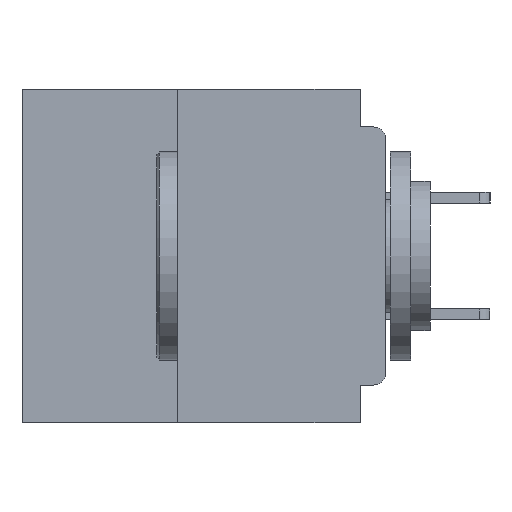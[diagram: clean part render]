
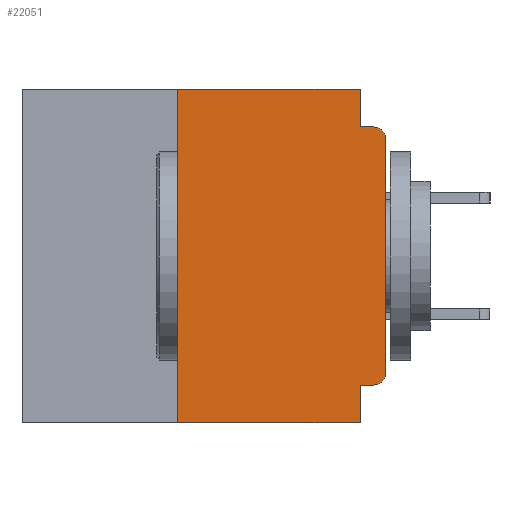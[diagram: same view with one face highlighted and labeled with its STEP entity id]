
A CAD part, left-side view. The second image highlights one B-rep face of the part: STEP entity #22051.
In plain terms, the highlighted planar face has unit normal (-1, 0, 0).
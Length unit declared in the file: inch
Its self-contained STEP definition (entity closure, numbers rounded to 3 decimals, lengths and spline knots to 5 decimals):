
#986 = ORIENTED_EDGE ( 'NONE', *, *, #8208, .F. ) ;
#1504 = EDGE_CURVE ( 'NONE', #35069, #13415, #29228, .T. ) ;
#2029 = VECTOR ( 'NONE', #14272, 39.37008 ) ;
#3005 = ORIENTED_EDGE ( 'NONE', *, *, #14251, .T. ) ;
#3397 = EDGE_LOOP ( 'NONE', ( #20141, #14638, #27694, #10907, #6797, #986, #3005, #25987, #33728, #25254 ) ) ;
#3756 = EDGE_CURVE ( 'NONE', #24772, #30169, #9292, .T. ) ;
#4642 = EDGE_CURVE ( 'NONE', #4860, #24772, #22605, .T. ) ;
#4709 = CARTESIAN_POINT ( 'NONE',  ( 0., 0., -0.06 ) ) ;
#4860 = VERTEX_POINT ( 'NONE', #27530 ) ;
#6797 = ORIENTED_EDGE ( 'NONE', *, *, #12264, .F. ) ;
#6902 = VECTOR ( 'NONE', #32386, 39.37008 ) ;
#7118 = DIRECTION ( 'NONE',  ( 0., -1., 0. ) ) ;
#7163 = CARTESIAN_POINT ( 'NONE',  ( 0., 0.437, 0. ) ) ;
#7688 = VECTOR ( 'NONE', #7118, 39.37008 ) ;
#8208 = EDGE_CURVE ( 'NONE', #21292, #8969, #37492, .T. ) ;
#8738 = VECTOR ( 'NONE', #18260, 39.37008 ) ;
#8969 = VERTEX_POINT ( 'NONE', #14616 ) ;
#9292 = CIRCLE ( 'NONE', #12161, 0.015 ) ;
#9353 = CARTESIAN_POINT ( 'NONE',  ( 0., 0.015, -0.34 ) ) ;
#10907 = ORIENTED_EDGE ( 'NONE', *, *, #1504, .F. ) ;
#11303 = CARTESIAN_POINT ( 'NONE',  ( 0., 0., -0.355 ) ) ;
#11499 = DIRECTION ( 'NONE',  ( 0., -1., 0. ) ) ;
#12161 = AXIS2_PLACEMENT_3D ( 'NONE', #36863, #36502, #36310 ) ;
#12264 = EDGE_CURVE ( 'NONE', #8969, #35069, #24632, .T. ) ;
#12353 = DIRECTION ( 'NONE',  ( 0., 0., -1. ) ) ;
#13157 = EDGE_CURVE ( 'NONE', #33381, #4860, #26352, .T. ) ;
#13164 = DIRECTION ( 'NONE',  ( 0., 0., -1. ) ) ;
#13415 = VERTEX_POINT ( 'NONE', #13640 ) ;
#13640 = CARTESIAN_POINT ( 'NONE',  ( 0., 0.031, -0.045 ) ) ;
#13670 = VECTOR ( 'NONE', #23205, 39.37008 ) ;
#14251 = EDGE_CURVE ( 'NONE', #21292, #25386, #17182, .T. ) ;
#14272 = DIRECTION ( 'NONE',  ( 0., 1., 0. ) ) ;
#14616 = CARTESIAN_POINT ( 'NONE',  ( 0., 0.25, 0. ) ) ;
#14638 = ORIENTED_EDGE ( 'NONE', *, *, #3756, .T. ) ;
#15315 = CARTESIAN_POINT ( 'NONE',  ( 0., 0.031, -0.4 ) ) ;
#17182 = LINE ( 'NONE', #29037, #31638 ) ;
#17358 = CARTESIAN_POINT ( 'NONE',  ( 0., 0.437, 0. ) ) ;
#18260 = DIRECTION ( 'NONE',  ( 0., 0., -1. ) ) ;
#18282 = EDGE_CURVE ( 'NONE', #33282, #25386, #32060, .T. ) ;
#18931 = CARTESIAN_POINT ( 'NONE',  ( 0., 0., -0.045 ) ) ;
#19632 = EDGE_CURVE ( 'NONE', #13415, #30169, #31067, .T. ) ;
#20078 = DIRECTION ( 'NONE',  ( 0., 0., 1. ) ) ;
#20135 = CARTESIAN_POINT ( 'NONE',  ( 0., 0.031, -0.4 ) ) ;
#20141 = ORIENTED_EDGE ( 'NONE', *, *, #4642, .T. ) ;
#20206 = AXIS2_PLACEMENT_3D ( 'NONE', #7163, #30635, #13164 ) ;
#21292 = VERTEX_POINT ( 'NONE', #27016 ) ;
#22051 = ADVANCED_FACE ( 'NONE', ( #35755 ), #27736, .F. ) ;
#22605 = LINE ( 'NONE', #32009, #6902 ) ;
#23205 = DIRECTION ( 'NONE',  ( 0., 0., -1. ) ) ;
#23733 = VECTOR ( 'NONE', #28919, 39.37008 ) ;
#24256 = EDGE_CURVE ( 'NONE', #33381, #33282, #25670, .T. ) ;
#24632 = LINE ( 'NONE', #17358, #23733 ) ;
#24772 = VERTEX_POINT ( 'NONE', #4709 ) ;
#24796 = CARTESIAN_POINT ( 'NONE',  ( 0., 0.031, -0.355 ) ) ;
#25254 = ORIENTED_EDGE ( 'NONE', *, *, #13157, .T. ) ;
#25386 = VERTEX_POINT ( 'NONE', #20135 ) ;
#25670 = LINE ( 'NONE', #11303, #2029 ) ;
#25987 = ORIENTED_EDGE ( 'NONE', *, *, #18282, .F. ) ;
#26352 = CIRCLE ( 'NONE', #29706, 0.015 ) ;
#26623 = CARTESIAN_POINT ( 'NONE',  ( 0., 0.031, 0. ) ) ;
#27016 = CARTESIAN_POINT ( 'NONE',  ( 0., 0.25, -0.4 ) ) ;
#27530 = CARTESIAN_POINT ( 'NONE',  ( 0., 0., -0.34 ) ) ;
#27694 = ORIENTED_EDGE ( 'NONE', *, *, #19632, .F. ) ;
#27736 = PLANE ( 'NONE',  #20206 ) ;
#28701 = CARTESIAN_POINT ( 'NONE',  ( 0., 0.25, -0.4 ) ) ;
#28919 = DIRECTION ( 'NONE',  ( 0., -1., 0. ) ) ;
#29037 = CARTESIAN_POINT ( 'NONE',  ( 0., 0.437, -0.4 ) ) ;
#29228 = LINE ( 'NONE', #26623, #13670 ) ;
#29706 = AXIS2_PLACEMENT_3D ( 'NONE', #9353, #29870, #12353 ) ;
#29870 = DIRECTION ( 'NONE',  ( -1., 0., 0. ) ) ;
#30051 = VECTOR ( 'NONE', #20078, 39.37008 ) ;
#30169 = VERTEX_POINT ( 'NONE', #35714 ) ;
#30613 = CARTESIAN_POINT ( 'NONE',  ( 0., 0.031, 0. ) ) ;
#30635 = DIRECTION ( 'NONE',  ( 1., 0., 0. ) ) ;
#31067 = LINE ( 'NONE', #18931, #7688 ) ;
#31638 = VECTOR ( 'NONE', #11499, 39.37008 ) ;
#32009 = CARTESIAN_POINT ( 'NONE',  ( 0., 0., 0. ) ) ;
#32060 = LINE ( 'NONE', #15315, #8738 ) ;
#32386 = DIRECTION ( 'NONE',  ( 0., 0., 1. ) ) ;
#33282 = VERTEX_POINT ( 'NONE', #24796 ) ;
#33381 = VERTEX_POINT ( 'NONE', #36470 ) ;
#33728 = ORIENTED_EDGE ( 'NONE', *, *, #24256, .F. ) ;
#35069 = VERTEX_POINT ( 'NONE', #30613 ) ;
#35714 = CARTESIAN_POINT ( 'NONE',  ( 0., 0.015, -0.045 ) ) ;
#35755 = FACE_OUTER_BOUND ( 'NONE', #3397, .T. ) ;
#36310 = DIRECTION ( 'NONE',  ( 0., 0., -1. ) ) ;
#36470 = CARTESIAN_POINT ( 'NONE',  ( 0., 0.015, -0.355 ) ) ;
#36502 = DIRECTION ( 'NONE',  ( -1., 0., 0. ) ) ;
#36863 = CARTESIAN_POINT ( 'NONE',  ( 0., 0.015, -0.06 ) ) ;
#37492 = LINE ( 'NONE', #28701, #30051 ) ;
